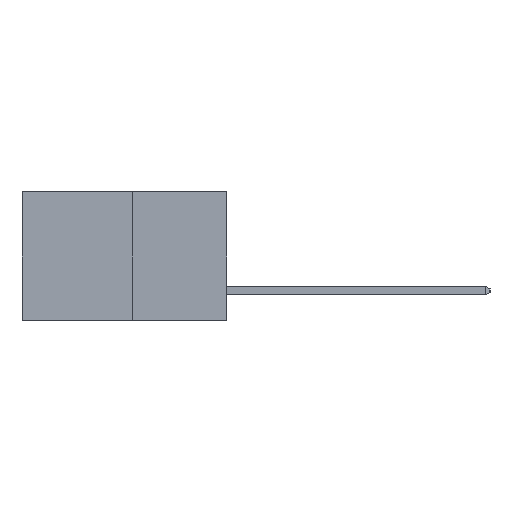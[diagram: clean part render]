
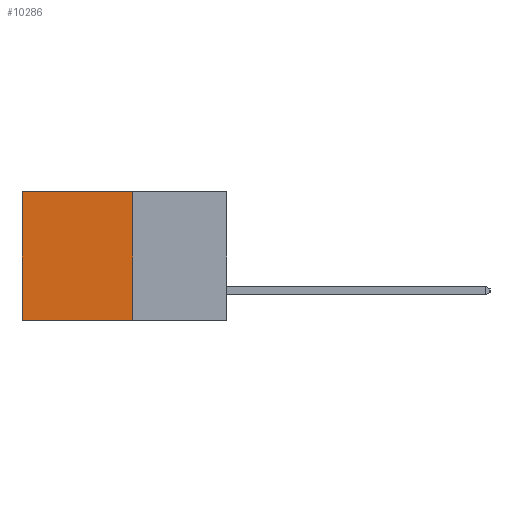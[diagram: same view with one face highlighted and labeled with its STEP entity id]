
A CAD part, left-side view. The second image highlights one B-rep face of the part: STEP entity #10286.
In plain terms, the highlighted planar face has unit normal (-1, 0, 0).
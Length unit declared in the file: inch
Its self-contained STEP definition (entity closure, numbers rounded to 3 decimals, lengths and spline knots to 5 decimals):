
#137 = CARTESIAN_POINT ( 'NONE',  ( 0.277, 0.27, -0.37 ) ) ;
#610 = LINE ( 'NONE', #5923, #12793 ) ;
#674 = LINE ( 'NONE', #11968, #3463 ) ;
#1044 = EDGE_CURVE ( 'NONE', #7985, #8685, #9845, .T. ) ;
#1321 = FACE_OUTER_BOUND ( 'NONE', #3036, .T. ) ;
#2456 = VERTEX_POINT ( 'NONE', #12368 ) ;
#2517 = CARTESIAN_POINT ( 'NONE',  ( 0.277, 0.27, 0. ) ) ;
#2535 = DIRECTION ( 'NONE',  ( 0., 1., 0. ) ) ;
#3036 = EDGE_LOOP ( 'NONE', ( #13170, #14087, #6282, #3897 ) ) ;
#3463 = VECTOR ( 'NONE', #2535, 39.37008 ) ;
#3808 = CARTESIAN_POINT ( 'NONE',  ( 0.277, 0.27, -0.37 ) ) ;
#3897 = ORIENTED_EDGE ( 'NONE', *, *, #13145, .T. ) ;
#4545 = LINE ( 'NONE', #14007, #7331 ) ;
#4676 = DIRECTION ( 'NONE',  ( 0., 0., -1. ) ) ;
#5028 = DIRECTION ( 'NONE',  ( 0., 0., -1. ) ) ;
#5923 = CARTESIAN_POINT ( 'NONE',  ( 0.277, 0.27, -0.37 ) ) ;
#6282 = ORIENTED_EDGE ( 'NONE', *, *, #1044, .F. ) ;
#6697 = VECTOR ( 'NONE', #7825, 39.37008 ) ;
#7286 = VERTEX_POINT ( 'NONE', #14172 ) ;
#7331 = VECTOR ( 'NONE', #4676, 39.37008 ) ;
#7825 = DIRECTION ( 'NONE',  ( 0., 0., -1. ) ) ;
#7985 = VERTEX_POINT ( 'NONE', #2517 ) ;
#8300 = DIRECTION ( 'NONE',  ( 0., 1., 0. ) ) ;
#8517 = PLANE ( 'NONE',  #12300 ) ;
#8685 = VERTEX_POINT ( 'NONE', #137 ) ;
#9459 = EDGE_CURVE ( 'NONE', #7286, #2456, #4545, .T. ) ;
#9489 = EDGE_CURVE ( 'NONE', #8685, #2456, #610, .T. ) ;
#9845 = LINE ( 'NONE', #12723, #6697 ) ;
#10286 = ADVANCED_FACE ( 'NONE', ( #1321 ), #8517, .F. ) ;
#11968 = CARTESIAN_POINT ( 'NONE',  ( 0.277, 0.27, 0. ) ) ;
#12030 = DIRECTION ( 'NONE',  ( 1., 0., 0. ) ) ;
#12300 = AXIS2_PLACEMENT_3D ( 'NONE', #3808, #12030, #5028 ) ;
#12368 = CARTESIAN_POINT ( 'NONE',  ( 0.277, 0.59, -0.37 ) ) ;
#12723 = CARTESIAN_POINT ( 'NONE',  ( 0.277, 0.27, -0.37 ) ) ;
#12793 = VECTOR ( 'NONE', #8300, 39.37008 ) ;
#13145 = EDGE_CURVE ( 'NONE', #7985, #7286, #674, .T. ) ;
#13170 = ORIENTED_EDGE ( 'NONE', *, *, #9459, .T. ) ;
#14007 = CARTESIAN_POINT ( 'NONE',  ( 0.277, 0.59, -0.37 ) ) ;
#14087 = ORIENTED_EDGE ( 'NONE', *, *, #9489, .F. ) ;
#14172 = CARTESIAN_POINT ( 'NONE',  ( 0.277, 0.59, 0. ) ) ;
